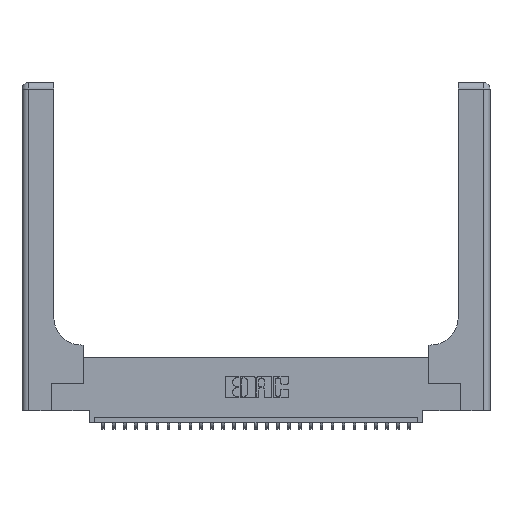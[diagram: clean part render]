
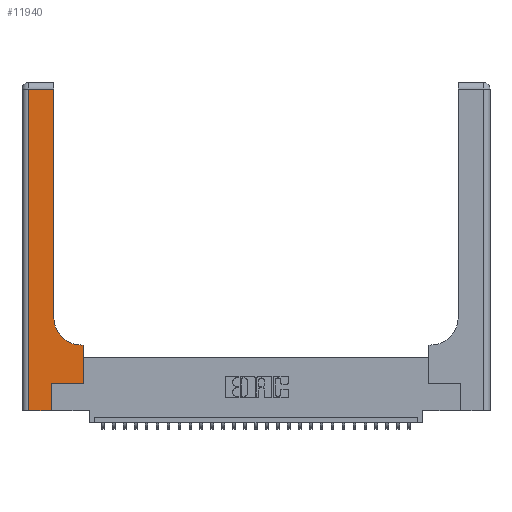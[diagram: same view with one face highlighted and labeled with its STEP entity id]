
A CAD part, top view. The second image highlights one B-rep face of the part: STEP entity #11940.
In plain terms, the highlighted planar face has unit normal (0, 0, 1).
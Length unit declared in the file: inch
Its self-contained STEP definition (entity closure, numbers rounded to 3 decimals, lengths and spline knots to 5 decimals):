
#248 = EDGE_CURVE ( 'NONE', #24819, #3854, #22625, .T. ) ;
#862 = CARTESIAN_POINT ( 'NONE',  ( 0., 2.94, 0.37 ) ) ;
#2238 = VERTEX_POINT ( 'NONE', #6385 ) ;
#2321 = LINE ( 'NONE', #26539, #12130 ) ;
#2533 = ORIENTED_EDGE ( 'NONE', *, *, #27076, .T. ) ;
#3040 = CARTESIAN_POINT ( 'NONE',  ( 0.2915, 0.85, 0.37 ) ) ;
#3137 = ORIENTED_EDGE ( 'NONE', *, *, #4929, .T. ) ;
#3757 = EDGE_CURVE ( 'NONE', #18251, #22670, #19090, .T. ) ;
#3854 = VERTEX_POINT ( 'NONE', #16246 ) ;
#4309 = VECTOR ( 'NONE', #14560, 39.37008 ) ;
#4481 = ORIENTED_EDGE ( 'NONE', *, *, #3757, .T. ) ;
#4881 = DIRECTION ( 'NONE',  ( 0., 1., 0. ) ) ;
#4908 = AXIS2_PLACEMENT_3D ( 'NONE', #10847, #8286, #8384 ) ;
#4929 = EDGE_CURVE ( 'NONE', #3854, #6419, #9560, .T. ) ;
#5083 = AXIS2_PLACEMENT_3D ( 'NONE', #16905, #28651, #15317 ) ;
#5411 = CARTESIAN_POINT ( 'NONE',  ( 0.2915, 0.6, 0.37 ) ) ;
#5723 = VECTOR ( 'NONE', #20905, 39.37008 ) ;
#6385 = CARTESIAN_POINT ( 'NONE',  ( 0.269, 0.25, 0.37 ) ) ;
#6419 = VERTEX_POINT ( 'NONE', #26490 ) ;
#6538 = ORIENTED_EDGE ( 'NONE', *, *, #18872, .T. ) ;
#6701 = EDGE_CURVE ( 'NONE', #10240, #24819, #15029, .T. ) ;
#8286 = DIRECTION ( 'NONE',  ( 0., 0., -1. ) ) ;
#8361 = VECTOR ( 'NONE', #4881, 39.37008 ) ;
#8384 = DIRECTION ( 'NONE',  ( -1., 0., 0. ) ) ;
#8503 = ORIENTED_EDGE ( 'NONE', *, *, #248, .T. ) ;
#9257 = ORIENTED_EDGE ( 'NONE', *, *, #6701, .T. ) ;
#9560 = LINE ( 'NONE', #27921, #4309 ) ;
#10240 = VERTEX_POINT ( 'NONE', #19372 ) ;
#10847 = CARTESIAN_POINT ( 'NONE',  ( 0., 3., 0.37 ) ) ;
#10891 = ORIENTED_EDGE ( 'NONE', *, *, #12052, .T. ) ;
#11105 = DIRECTION ( 'NONE',  ( 1., 0., 0. ) ) ;
#11310 = EDGE_CURVE ( 'NONE', #2238, #18251, #22803, .T. ) ;
#11708 = CARTESIAN_POINT ( 'NONE',  ( 0.5585, 0.25, 0.37 ) ) ;
#11940 = ADVANCED_FACE ( 'NONE', ( #25588 ), #21742, .F. ) ;
#12051 = CARTESIAN_POINT ( 'NONE',  ( 0.06, 2.94, 0.37 ) ) ;
#12052 = EDGE_CURVE ( 'NONE', #22251, #10240, #12928, .T. ) ;
#12130 = VECTOR ( 'NONE', #13069, 39.37008 ) ;
#12928 = LINE ( 'NONE', #18276, #8361 ) ;
#13069 = DIRECTION ( 'NONE',  ( 0., 1., 0. ) ) ;
#13782 = EDGE_CURVE ( 'NONE', #6419, #2238, #2321, .T. ) ;
#14560 = DIRECTION ( 'NONE',  ( 1., 0., 0. ) ) ;
#15029 = LINE ( 'NONE', #862, #24560 ) ;
#15317 = DIRECTION ( 'NONE',  ( 1., 0., 0. ) ) ;
#15366 = CARTESIAN_POINT ( 'NONE',  ( 0.5585, 0.25, 0.37 ) ) ;
#15966 = CARTESIAN_POINT ( 'NONE',  ( 0.06, 3., 0.37 ) ) ;
#16246 = CARTESIAN_POINT ( 'NONE',  ( 0.06, 0., 0.37 ) ) ;
#16905 = CARTESIAN_POINT ( 'NONE',  ( 0.5415, 0.85, 0.37 ) ) ;
#17190 = CARTESIAN_POINT ( 'NONE',  ( 0.269, 0.25, 0.37 ) ) ;
#18251 = VERTEX_POINT ( 'NONE', #11708 ) ;
#18276 = CARTESIAN_POINT ( 'NONE',  ( 0.2915, 3., 0.37 ) ) ;
#18658 = LINE ( 'NONE', #5411, #22900 ) ;
#18872 = EDGE_CURVE ( 'NONE', #22670, #23207, #18658, .T. ) ;
#18980 = ORIENTED_EDGE ( 'NONE', *, *, #11310, .T. ) ;
#19090 = LINE ( 'NONE', #15366, #5723 ) ;
#19372 = CARTESIAN_POINT ( 'NONE',  ( 0.2915, 2.94, 0.37 ) ) ;
#19470 = VECTOR ( 'NONE', #27366, 39.37008 ) ;
#20222 = CARTESIAN_POINT ( 'NONE',  ( 0.5585, 0.6, 0.37 ) ) ;
#20905 = DIRECTION ( 'NONE',  ( 0., 1., 0. ) ) ;
#21742 = PLANE ( 'NONE',  #4908 ) ;
#22251 = VERTEX_POINT ( 'NONE', #3040 ) ;
#22392 = CIRCLE ( 'NONE', #5083, 0.25 ) ;
#22625 = LINE ( 'NONE', #15966, #19470 ) ;
#22670 = VERTEX_POINT ( 'NONE', #20222 ) ;
#22803 = LINE ( 'NONE', #17190, #27710 ) ;
#22900 = VECTOR ( 'NONE', #23380, 39.37008 ) ;
#23207 = VERTEX_POINT ( 'NONE', #28629 ) ;
#23380 = DIRECTION ( 'NONE',  ( -1., 0., 0. ) ) ;
#24560 = VECTOR ( 'NONE', #25333, 39.37008 ) ;
#24819 = VERTEX_POINT ( 'NONE', #12051 ) ;
#25333 = DIRECTION ( 'NONE',  ( -1., 0., 0. ) ) ;
#25353 = ORIENTED_EDGE ( 'NONE', *, *, #13782, .T. ) ;
#25369 = EDGE_LOOP ( 'NONE', ( #10891, #9257, #8503, #3137, #25353, #18980, #4481, #6538, #2533 ) ) ;
#25588 = FACE_OUTER_BOUND ( 'NONE', #25369, .T. ) ;
#26490 = CARTESIAN_POINT ( 'NONE',  ( 0.269, 0., 0.37 ) ) ;
#26539 = CARTESIAN_POINT ( 'NONE',  ( 0.269, 0., 0.37 ) ) ;
#27076 = EDGE_CURVE ( 'NONE', #23207, #22251, #22392, .T. ) ;
#27366 = DIRECTION ( 'NONE',  ( 0., -1., 0. ) ) ;
#27710 = VECTOR ( 'NONE', #11105, 39.37008 ) ;
#27921 = CARTESIAN_POINT ( 'NONE',  ( 0., 0., 0.37 ) ) ;
#28629 = CARTESIAN_POINT ( 'NONE',  ( 0.5415, 0.6, 0.37 ) ) ;
#28651 = DIRECTION ( 'NONE',  ( 0., 0., -1. ) ) ;
